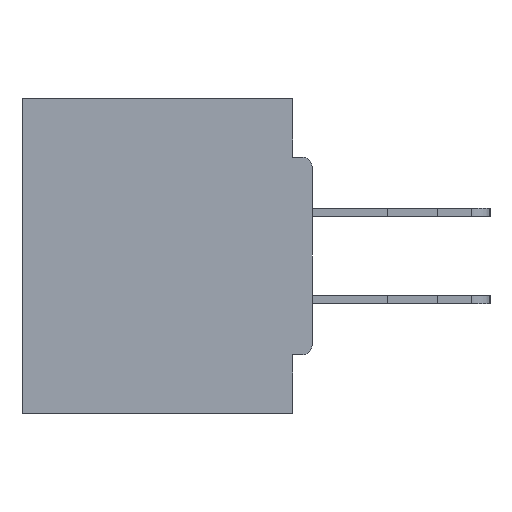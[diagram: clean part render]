
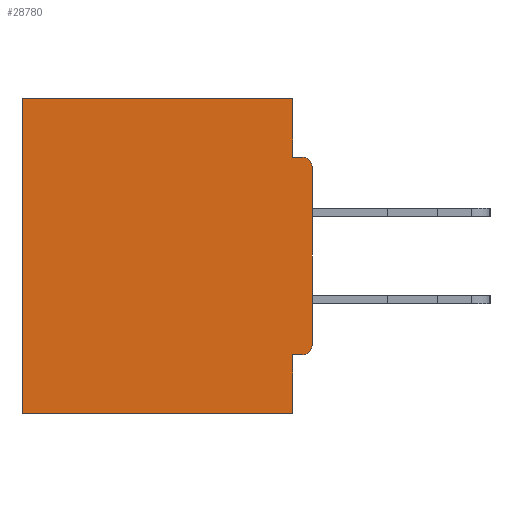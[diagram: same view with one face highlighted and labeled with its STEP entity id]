
A CAD part, left-side view. The second image highlights one B-rep face of the part: STEP entity #28780.
In plain terms, the highlighted planar face has unit normal (-1, 0, 0).
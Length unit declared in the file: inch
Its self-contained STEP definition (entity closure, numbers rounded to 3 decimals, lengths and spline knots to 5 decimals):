
#549 = CIRCLE ( 'NONE', #3236, 0.015 ) ;
#975 = CARTESIAN_POINT ( 'NONE',  ( 0.298, 0., -0.1085 ) ) ;
#1114 = CARTESIAN_POINT ( 'NONE',  ( 0.298, 0.031, -0.5 ) ) ;
#1138 = DIRECTION ( 'NONE',  ( 0., -1., 0. ) ) ;
#1877 = CARTESIAN_POINT ( 'NONE',  ( 0.298, 0., -0.3915 ) ) ;
#1992 = DIRECTION ( 'NONE',  ( -1., 0., 0. ) ) ;
#2828 = ORIENTED_EDGE ( 'NONE', *, *, #5886, .F. ) ;
#2989 = EDGE_CURVE ( 'NONE', #29093, #36352, #30802, .T. ) ;
#3114 = CARTESIAN_POINT ( 'NONE',  ( 0.298, 0., 0. ) ) ;
#3155 = VECTOR ( 'NONE', #13212, 39.37008 ) ;
#3236 = AXIS2_PLACEMENT_3D ( 'NONE', #10635, #1992, #10764 ) ;
#4443 = CARTESIAN_POINT ( 'NONE',  ( 0.298, 0.031, 0. ) ) ;
#4712 = EDGE_CURVE ( 'NONE', #32692, #11709, #27052, .T. ) ;
#4930 = VERTEX_POINT ( 'NONE', #975 ) ;
#5143 = DIRECTION ( 'NONE',  ( 0., 1., 0. ) ) ;
#5387 = ORIENTED_EDGE ( 'NONE', *, *, #23858, .F. ) ;
#5744 = VECTOR ( 'NONE', #14430, 39.37008 ) ;
#5886 = EDGE_CURVE ( 'NONE', #6376, #32692, #23699, .T. ) ;
#6263 = PLANE ( 'NONE',  #12267 ) ;
#6376 = VERTEX_POINT ( 'NONE', #25780 ) ;
#6702 = AXIS2_PLACEMENT_3D ( 'NONE', #15556, #15788, #15682 ) ;
#6917 = CARTESIAN_POINT ( 'NONE',  ( 0.298, 0.46, 0. ) ) ;
#7126 = VECTOR ( 'NONE', #7947, 39.37008 ) ;
#7542 = EDGE_CURVE ( 'NONE', #15707, #18375, #16732, .T. ) ;
#7947 = DIRECTION ( 'NONE',  ( 0., 0., -1. ) ) ;
#8654 = LINE ( 'NONE', #24722, #3155 ) ;
#8739 = EDGE_CURVE ( 'NONE', #29093, #17238, #18006, .T. ) ;
#9204 = DIRECTION ( 'NONE',  ( 1., 0., 0. ) ) ;
#10635 = CARTESIAN_POINT ( 'NONE',  ( 0.298, 0.015, -0.1085 ) ) ;
#10764 = DIRECTION ( 'NONE',  ( 0., 0., -1. ) ) ;
#11616 = ORIENTED_EDGE ( 'NONE', *, *, #4712, .F. ) ;
#11709 = VERTEX_POINT ( 'NONE', #19117 ) ;
#11742 = CARTESIAN_POINT ( 'NONE',  ( 0.298, 0., 0. ) ) ;
#12267 = AXIS2_PLACEMENT_3D ( 'NONE', #11742, #9204, #23365 ) ;
#13212 = DIRECTION ( 'NONE',  ( 0., 0., -1. ) ) ;
#14430 = DIRECTION ( 'NONE',  ( 0., 1., 0. ) ) ;
#14631 = VECTOR ( 'NONE', #1138, 39.37008 ) ;
#15556 = CARTESIAN_POINT ( 'NONE',  ( 0.298, 0.015, -0.3915 ) ) ;
#15682 = DIRECTION ( 'NONE',  ( 0., 0., -1. ) ) ;
#15707 = VERTEX_POINT ( 'NONE', #35964 ) ;
#15788 = DIRECTION ( 'NONE',  ( -1., 0., 0. ) ) ;
#16732 = CIRCLE ( 'NONE', #6702, 0.015 ) ;
#16742 = ORIENTED_EDGE ( 'NONE', *, *, #27874, .T. ) ;
#16975 = CARTESIAN_POINT ( 'NONE',  ( 0.298, 0.031, -0.5 ) ) ;
#17202 = CARTESIAN_POINT ( 'NONE',  ( 0.298, 0., -0.5 ) ) ;
#17238 = VERTEX_POINT ( 'NONE', #33643 ) ;
#18006 = LINE ( 'NONE', #1114, #23871 ) ;
#18234 = VERTEX_POINT ( 'NONE', #29304 ) ;
#18375 = VERTEX_POINT ( 'NONE', #1877 ) ;
#19117 = CARTESIAN_POINT ( 'NONE',  ( 0.298, 0.46, -0.5 ) ) ;
#19373 = ORIENTED_EDGE ( 'NONE', *, *, #23791, .F. ) ;
#19712 = CARTESIAN_POINT ( 'NONE',  ( 0.298, 0., 0. ) ) ;
#20467 = ORIENTED_EDGE ( 'NONE', *, *, #7542, .T. ) ;
#21238 = ORIENTED_EDGE ( 'NONE', *, *, #8739, .F. ) ;
#21395 = DIRECTION ( 'NONE',  ( 0., 0., -1. ) ) ;
#22035 = VECTOR ( 'NONE', #5143, 39.37008 ) ;
#23007 = DIRECTION ( 'NONE',  ( 0., 1., 0. ) ) ;
#23365 = DIRECTION ( 'NONE',  ( 0., 0., -1. ) ) ;
#23699 = LINE ( 'NONE', #24596, #36369 ) ;
#23791 = EDGE_CURVE ( 'NONE', #15707, #6376, #37431, .T. ) ;
#23858 = EDGE_CURVE ( 'NONE', #4930, #18375, #27958, .T. ) ;
#23871 = VECTOR ( 'NONE', #21395, 39.37008 ) ;
#24058 = CARTESIAN_POINT ( 'NONE',  ( 0.298, 0., -0.0935 ) ) ;
#24596 = CARTESIAN_POINT ( 'NONE',  ( 0.298, 0.031, -0.5 ) ) ;
#24722 = CARTESIAN_POINT ( 'NONE',  ( 0.298, 0.46, 0. ) ) ;
#25780 = CARTESIAN_POINT ( 'NONE',  ( 0.298, 0.031, -0.4065 ) ) ;
#26895 = LINE ( 'NONE', #24058, #14631 ) ;
#27052 = LINE ( 'NONE', #17202, #5744 ) ;
#27686 = EDGE_CURVE ( 'NONE', #17238, #18234, #26895, .T. ) ;
#27874 = EDGE_CURVE ( 'NONE', #4930, #18234, #549, .T. ) ;
#27958 = LINE ( 'NONE', #19712, #7126 ) ;
#28156 = DIRECTION ( 'NONE',  ( 0., 0., -1. ) ) ;
#28780 = ADVANCED_FACE ( 'NONE', ( #36703 ), #6263, .F. ) ;
#29032 = EDGE_CURVE ( 'NONE', #36352, #11709, #8654, .T. ) ;
#29093 = VERTEX_POINT ( 'NONE', #4443 ) ;
#29304 = CARTESIAN_POINT ( 'NONE',  ( 0.298, 0.015, -0.0935 ) ) ;
#30802 = LINE ( 'NONE', #3114, #31251 ) ;
#30867 = CARTESIAN_POINT ( 'NONE',  ( 0.298, 0., -0.4065 ) ) ;
#31251 = VECTOR ( 'NONE', #23007, 39.37008 ) ;
#31474 = ORIENTED_EDGE ( 'NONE', *, *, #27686, .F. ) ;
#32692 = VERTEX_POINT ( 'NONE', #16975 ) ;
#33643 = CARTESIAN_POINT ( 'NONE',  ( 0.298, 0.031, -0.0935 ) ) ;
#34226 = ORIENTED_EDGE ( 'NONE', *, *, #29032, .T. ) ;
#35500 = ORIENTED_EDGE ( 'NONE', *, *, #2989, .T. ) ;
#35761 = EDGE_LOOP ( 'NONE', ( #16742, #31474, #21238, #35500, #34226, #11616, #2828, #19373, #20467, #5387 ) ) ;
#35964 = CARTESIAN_POINT ( 'NONE',  ( 0.298, 0.015, -0.4065 ) ) ;
#36352 = VERTEX_POINT ( 'NONE', #6917 ) ;
#36369 = VECTOR ( 'NONE', #28156, 39.37008 ) ;
#36703 = FACE_OUTER_BOUND ( 'NONE', #35761, .T. ) ;
#37431 = LINE ( 'NONE', #30867, #22035 ) ;
